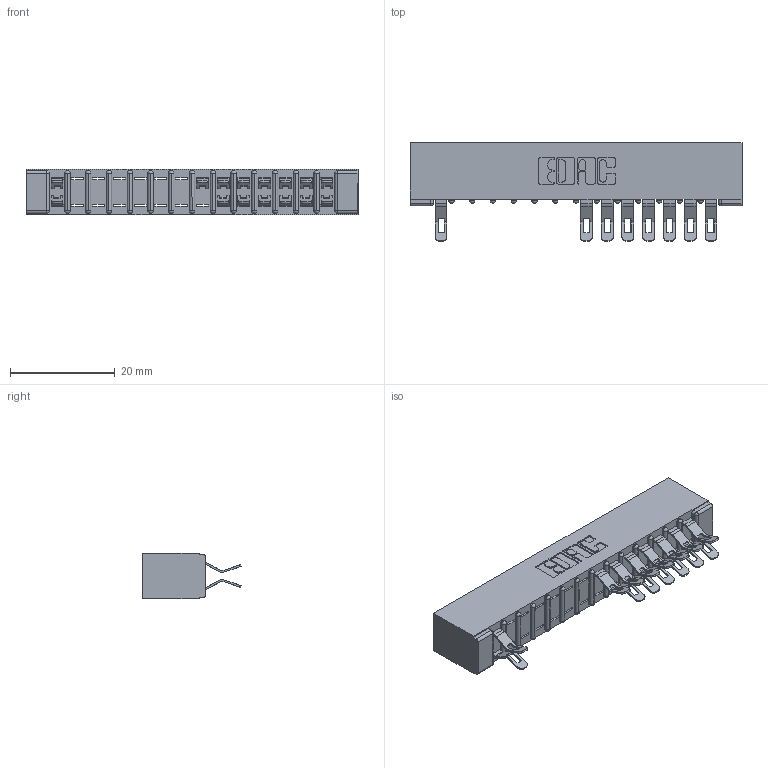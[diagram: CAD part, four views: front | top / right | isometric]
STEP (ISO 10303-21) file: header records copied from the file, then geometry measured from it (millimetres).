
FILE_DESCRIPTION (( 'STEP AP203' ), '1' );
FILE_NAME ('357-028-555-201.STEP', '2018-08-09T06:49:52', ( '' ), ( '' ), 'SwSTEP 2.0', 'SolidWorks 2016', '' );
FILE_SCHEMA (( 'CONFIG_CONTROL_DESIGN' ));
Length unit declared in the file: inch
Products named in the file (3): 357-028-555-201; 307 Part_No Mounting Lugs; 307-290-001_555
Assembly tree (16 placements, depth 2):
  357-028-555-201
    307 Part_No Mounting Lugs
    307-290-001_555  x15
Bounding box: 63.35 x 18.75 x 8.71 mm (x, y, z)
Volume: 4254 mm3; surface area: 6819.9 mm2
Topology: 16 solids, 16 shells, 1170 faces, 3430 edges, 2224 vertices
Faces by surface type: plane 654, cylinder 486, sphere 30
Entity records: 15745 total; most frequent: CARTESIAN_POINT 2641, ORIENTED_EDGE 2628, DIRECTION 2592, EDGE_CURVE 1314, VECTOR 986, LINE 986, VERTEX_POINT 852, AXIS2_PLACEMENT_3D 803
